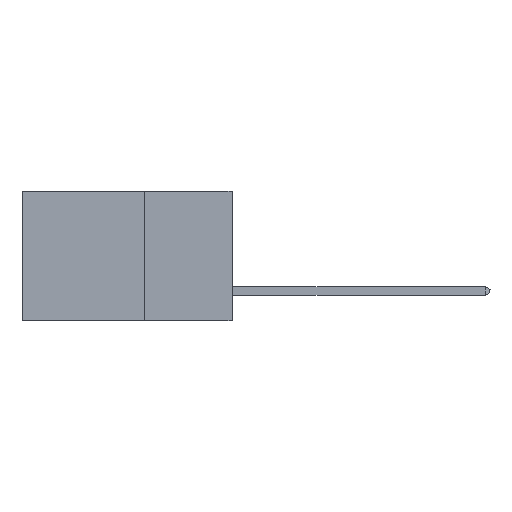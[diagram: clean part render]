
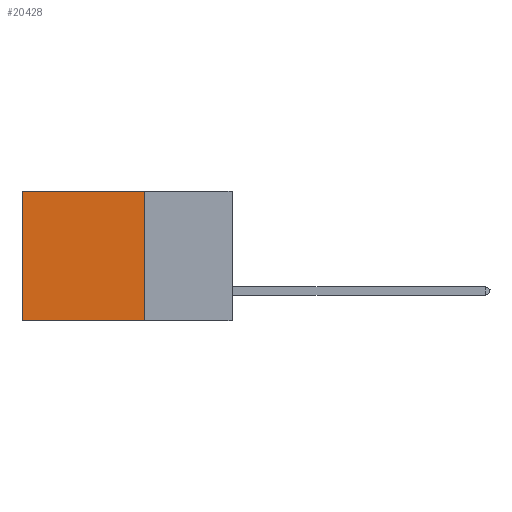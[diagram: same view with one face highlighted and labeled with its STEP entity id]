
A CAD part, left-side view. The second image highlights one B-rep face of the part: STEP entity #20428.
In plain terms, the highlighted planar face has unit normal (-1, 0, 0).
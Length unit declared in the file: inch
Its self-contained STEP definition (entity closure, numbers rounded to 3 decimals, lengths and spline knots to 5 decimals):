
#505 = VERTEX_POINT ( 'NONE', #3013 ) ;
#512 = CARTESIAN_POINT ( 'NONE',  ( 0.2875, 0.25, 0. ) ) ;
#1309 = CARTESIAN_POINT ( 'NONE',  ( 0.2875, 0.25, -0.37 ) ) ;
#1348 = FACE_OUTER_BOUND ( 'NONE', #15283, .T. ) ;
#2084 = CARTESIAN_POINT ( 'NONE',  ( 0.2875, 0.6, 0. ) ) ;
#2442 = CARTESIAN_POINT ( 'NONE',  ( 0.2875, 0.25, 0. ) ) ;
#3013 = CARTESIAN_POINT ( 'NONE',  ( 0.2875, 0.6, -0.37 ) ) ;
#3186 = LINE ( 'NONE', #13445, #9137 ) ;
#3574 = EDGE_CURVE ( 'NONE', #7807, #505, #3186, .T. ) ;
#3846 = DIRECTION ( 'NONE',  ( 0., 1., 0. ) ) ;
#3904 = DIRECTION ( 'NONE',  ( 0., 0., -1. ) ) ;
#4106 = VERTEX_POINT ( 'NONE', #14555 ) ;
#6510 = AXIS2_PLACEMENT_3D ( 'NONE', #8425, #23764, #18125 ) ;
#6771 = LINE ( 'NONE', #23849, #16429 ) ;
#7807 = VERTEX_POINT ( 'NONE', #1309 ) ;
#7855 = DIRECTION ( 'NONE',  ( 0., 1., 0. ) ) ;
#8425 = CARTESIAN_POINT ( 'NONE',  ( 0.2875, 0.25, 0. ) ) ;
#8528 = EDGE_CURVE ( 'NONE', #13631, #7807, #11631, .T. ) ;
#9137 = VECTOR ( 'NONE', #3846, 39.37008 ) ;
#9677 = VECTOR ( 'NONE', #3904, 39.37008 ) ;
#9778 = ORIENTED_EDGE ( 'NONE', *, *, #17721, .T. ) ;
#10075 = DIRECTION ( 'NONE',  ( 0., 0., -1. ) ) ;
#11631 = LINE ( 'NONE', #512, #17080 ) ;
#13445 = CARTESIAN_POINT ( 'NONE',  ( 0.2875, 0.25, -0.37 ) ) ;
#13631 = VERTEX_POINT ( 'NONE', #2442 ) ;
#14555 = CARTESIAN_POINT ( 'NONE',  ( 0.2875, 0.6, 0. ) ) ;
#15283 = EDGE_LOOP ( 'NONE', ( #22902, #21044, #23505, #9778 ) ) ;
#16429 = VECTOR ( 'NONE', #7855, 39.37008 ) ;
#17080 = VECTOR ( 'NONE', #10075, 39.37008 ) ;
#17721 = EDGE_CURVE ( 'NONE', #13631, #4106, #6771, .T. ) ;
#18125 = DIRECTION ( 'NONE',  ( 0., 0., -1. ) ) ;
#19021 = LINE ( 'NONE', #2084, #9677 ) ;
#20153 = EDGE_CURVE ( 'NONE', #4106, #505, #19021, .T. ) ;
#20428 = ADVANCED_FACE ( 'NONE', ( #1348 ), #22004, .F. ) ;
#21044 = ORIENTED_EDGE ( 'NONE', *, *, #3574, .F. ) ;
#22004 = PLANE ( 'NONE',  #6510 ) ;
#22902 = ORIENTED_EDGE ( 'NONE', *, *, #20153, .T. ) ;
#23505 = ORIENTED_EDGE ( 'NONE', *, *, #8528, .F. ) ;
#23764 = DIRECTION ( 'NONE',  ( 1., 0., 0. ) ) ;
#23849 = CARTESIAN_POINT ( 'NONE',  ( 0.2875, 0.25, 0. ) ) ;
